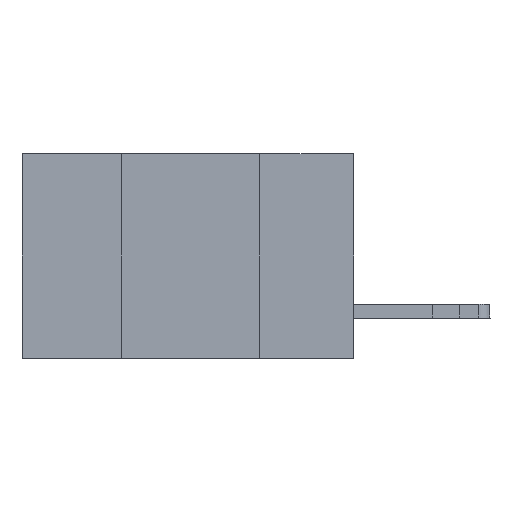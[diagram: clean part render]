
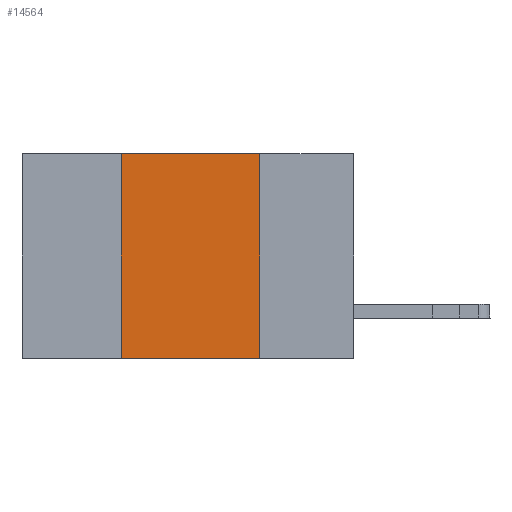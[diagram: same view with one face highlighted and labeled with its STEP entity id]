
A CAD part, left-side view. The second image highlights one B-rep face of the part: STEP entity #14564.
In plain terms, the highlighted planar face has unit normal (-1, 0, 0).
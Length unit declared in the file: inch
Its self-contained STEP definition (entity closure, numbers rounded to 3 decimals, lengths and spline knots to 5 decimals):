
#27 = EDGE_LOOP ( 'NONE', ( #27684, #14939, #6224, #15822 ) ) ;
#518 = VERTEX_POINT ( 'NONE', #19892 ) ;
#878 = VERTEX_POINT ( 'NONE', #24053 ) ;
#1434 = LINE ( 'NONE', #8092, #20750 ) ;
#1629 = PLANE ( 'NONE',  #22558 ) ;
#1647 = VERTEX_POINT ( 'NONE', #6565 ) ;
#3525 = FACE_OUTER_BOUND ( 'NONE', #27, .T. ) ;
#3582 = EDGE_CURVE ( 'NONE', #1647, #878, #16033, .T. ) ;
#5061 = EDGE_CURVE ( 'NONE', #16339, #518, #1434, .T. ) ;
#5543 = DIRECTION ( 'NONE',  ( 0., -1., 0. ) ) ;
#6224 = ORIENTED_EDGE ( 'NONE', *, *, #5061, .F. ) ;
#6565 = CARTESIAN_POINT ( 'NONE',  ( 0., 0.17, 0. ) ) ;
#8092 = CARTESIAN_POINT ( 'NONE',  ( 0., 0.42, 0. ) ) ;
#8343 = CARTESIAN_POINT ( 'NONE',  ( 0., 0.42, -0.37 ) ) ;
#9660 = VECTOR ( 'NONE', #22676, 39.37008 ) ;
#12494 = DIRECTION ( 'NONE',  ( 0., 0., -1. ) ) ;
#13902 = VECTOR ( 'NONE', #5543, 39.37008 ) ;
#14564 = ADVANCED_FACE ( 'NONE', ( #3525 ), #1629, .F. ) ;
#14939 = ORIENTED_EDGE ( 'NONE', *, *, #22010, .F. ) ;
#15822 = ORIENTED_EDGE ( 'NONE', *, *, #27911, .T. ) ;
#16033 = LINE ( 'NONE', #27410, #9660 ) ;
#16339 = VERTEX_POINT ( 'NONE', #8343 ) ;
#16702 = CARTESIAN_POINT ( 'NONE',  ( 0., 0.6, -0.37 ) ) ;
#17578 = CARTESIAN_POINT ( 'NONE',  ( 0., 0.6, 0. ) ) ;
#19151 = LINE ( 'NONE', #16702, #13902 ) ;
#19282 = DIRECTION ( 'NONE',  ( 1., 0., 0. ) ) ;
#19892 = CARTESIAN_POINT ( 'NONE',  ( 0., 0.42, 0. ) ) ;
#20750 = VECTOR ( 'NONE', #21402, 39.37008 ) ;
#21402 = DIRECTION ( 'NONE',  ( 0., 0., 1. ) ) ;
#21455 = CARTESIAN_POINT ( 'NONE',  ( 0., 0.6, 0. ) ) ;
#22010 = EDGE_CURVE ( 'NONE', #518, #1647, #28242, .T. ) ;
#22326 = VECTOR ( 'NONE', #23679, 39.37008 ) ;
#22558 = AXIS2_PLACEMENT_3D ( 'NONE', #21455, #19282, #12494 ) ;
#22676 = DIRECTION ( 'NONE',  ( 0., 0., -1. ) ) ;
#23679 = DIRECTION ( 'NONE',  ( 0., -1., 0. ) ) ;
#24053 = CARTESIAN_POINT ( 'NONE',  ( 0., 0.17, -0.37 ) ) ;
#27410 = CARTESIAN_POINT ( 'NONE',  ( 0., 0.17, 0. ) ) ;
#27684 = ORIENTED_EDGE ( 'NONE', *, *, #3582, .F. ) ;
#27911 = EDGE_CURVE ( 'NONE', #16339, #878, #19151, .T. ) ;
#28242 = LINE ( 'NONE', #17578, #22326 ) ;
